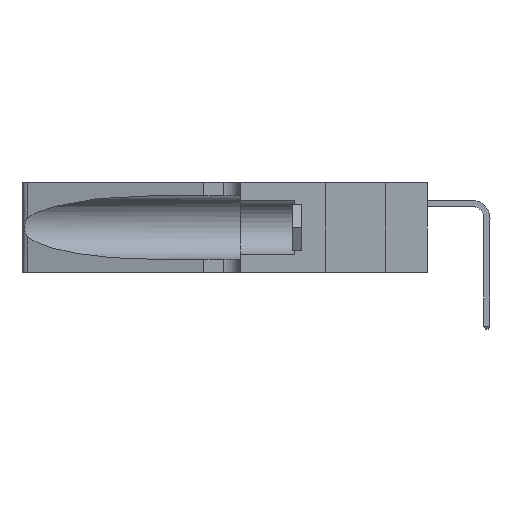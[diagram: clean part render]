
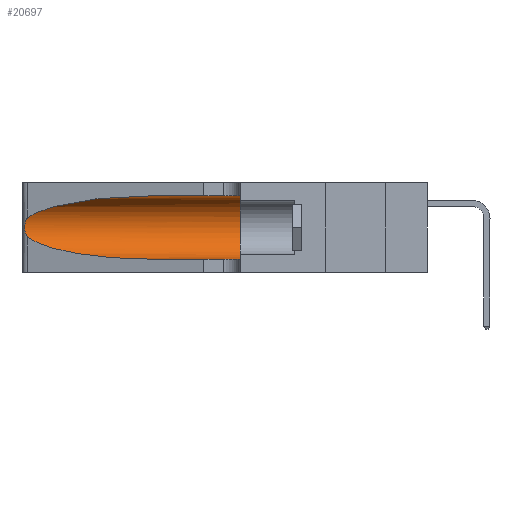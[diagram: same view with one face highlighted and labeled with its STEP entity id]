
A CAD part, left-side view. The second image highlights one B-rep face of the part: STEP entity #20697.
In plain terms, the highlighted cylindrical face has radius 3.308 mm (diameter 6.617 mm), a partial arc.
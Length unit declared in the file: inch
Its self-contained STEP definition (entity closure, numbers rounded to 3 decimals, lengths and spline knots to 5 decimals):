
#580 = VERTEX_POINT ( 'NONE', #30135 ) ;
#878 = VERTEX_POINT ( 'NONE', #23582 ) ;
#1025 = LINE ( 'NONE', #15702, #28114 ) ;
#1198 = DIRECTION ( 'NONE',  ( 0., 0., 1. ) ) ;
#1625 = CARTESIAN_POINT ( 'NONE',  ( 0.25787, 1.23484, 0.2124 ) ) ;
#4258 = CARTESIAN_POINT ( 'NONE',  ( 0.26018, 1.23835, 0.19895 ) ) ;
#4558 = CARTESIAN_POINT ( 'NONE',  ( 0.18966, 0.96281, 0.31525 ) ) ;
#4931 = EDGE_CURVE ( 'NONE', #878, #22970, #25974, .T. ) ;
#5900 = CIRCLE ( 'NONE', #28932, 0.13025 ) ;
#6622 = CYLINDRICAL_SURFACE ( 'NONE', #29486, 0.13025 ) ;
#6791 = CARTESIAN_POINT ( 'NONE',  ( 0.25555, 1.22994, 0.2215 ) ) ;
#6894 = CARTESIAN_POINT ( 'NONE',  ( 0.26075, 1.23896, 0.178 ) ) ;
#7195 = CARTESIAN_POINT ( 'NONE',  ( 0.2373, 1.15595, 0.28018 ) ) ;
#7427 = B_SPLINE_CURVE_WITH_KNOTS ( 'NONE', 3,
 ( #14649, #6791, #17309, #1625, #19964, #4258, #22632, #6894, #25282, #9506, #27890, #12143, #30555, #14763 ),
 .UNSPECIFIED., .F., .F.,
 ( 4, 2, 2, 2, 2, 2, 4 ),
 ( 0., 0.00027, 0.00053, 0.00107, 0.0016, 0.00187, 0.00214 ),
 .UNSPECIFIED. ) ;
#7447 = FACE_OUTER_BOUND ( 'NONE', #32667, .T. ) ;
#7489 = CARTESIAN_POINT ( 'NONE',  ( 0.2373, 1.15595, 0.08982 ) ) ;
#7947 = ORIENTED_EDGE ( 'NONE', *, *, #4931, .T. ) ;
#8421 = DIRECTION ( 'NONE',  ( 0., -1., 0. ) ) ;
#9506 = CARTESIAN_POINT ( 'NONE',  ( 0.25856, 1.23593, 0.16098 ) ) ;
#9768 = CARTESIAN_POINT ( 'NONE',  ( 0.1305, 1.61858, 0.185 ) ) ;
#10685 = CARTESIAN_POINT ( 'NONE',  ( 0.1305, 0.72297, 0.31525 ) ) ;
#12143 = CARTESIAN_POINT ( 'NONE',  ( 0.25639, 1.23186, 0.15144 ) ) ;
#12635 = CARTESIAN_POINT ( 'NONE',  ( 0.1305, 0.35, 0.31525 ) ) ;
#14649 = CARTESIAN_POINT ( 'NONE',  ( 0.25487, 1.22718, 0.22369 ) ) ;
#14763 = CARTESIAN_POINT ( 'NONE',  ( 0.25487, 1.22718, 0.14631 ) ) ;
#15386 = CARTESIAN_POINT ( 'NONE',  ( 0.1305, 0.72297, 0.05475 ) ) ;
#15601 = ORIENTED_EDGE ( 'NONE', *, *, #25103, .T. ) ;
#15702 = CARTESIAN_POINT ( 'NONE',  ( 0.1305, 1.61858, 0.31525 ) ) ;
#16545 = EDGE_CURVE ( 'NONE', #31386, #26524, #1025, .T. ) ;
#16882 = DIRECTION ( 'NONE',  ( 0., 1., 0. ) ) ;
#17309 = CARTESIAN_POINT ( 'NONE',  ( 0.25639, 1.23184, 0.21858 ) ) ;
#18256 = EDGE_CURVE ( 'NONE', #22970, #32600, #22673, .T. ) ;
#19964 = CARTESIAN_POINT ( 'NONE',  ( 0.25854, 1.2359, 0.20912 ) ) ;
#20272 = CARTESIAN_POINT ( 'NONE',  ( 0.1305, 0.72297, 0.31525 ) ) ;
#20697 = ADVANCED_FACE ( 'NONE', ( #7447 ), #6622, .F. ) ;
#22632 = CARTESIAN_POINT ( 'NONE',  ( 0.26075, 1.23896, 0.19203 ) ) ;
#22673 = LINE ( 'NONE', #24180, #30478 ) ;
#22970 = VERTEX_POINT ( 'NONE', #32320 ) ;
#23582 = CARTESIAN_POINT ( 'NONE',  ( 0.25487, 1.22718, 0.14631 ) ) ;
#24180 = CARTESIAN_POINT ( 'NONE',  ( 0.1305, 1.61858, 0.05475 ) ) ;
#24981 = ORIENTED_EDGE ( 'NONE', *, *, #27028, .T. ) ;
#25103 = EDGE_CURVE ( 'NONE', #31386, #580, #30370, .T. ) ;
#25282 = CARTESIAN_POINT ( 'NONE',  ( 0.26017, 1.23833, 0.17102 ) ) ;
#25534 = DIRECTION ( 'NONE',  ( 0., 0., -1. ) ) ;
#25561 = EDGE_CURVE ( 'NONE', #26524, #32600, #5900, .T. ) ;
#25581 = CARTESIAN_POINT ( 'NONE',  ( 0.25487, 1.22718, 0.22369 ) ) ;
#25974 =( BOUNDED_CURVE ( )  B_SPLINE_CURVE ( 3, ( #28376, #7489, #31142, #15386 ),
 .UNSPECIFIED., .F., .F. ) 
 B_SPLINE_CURVE_WITH_KNOTS ( ( 4, 4 ),
 ( 3.44316, 4.71239 ),
 .UNSPECIFIED. ) 
 CURVE ( )  GEOMETRIC_REPRESENTATION_ITEM ( )  RATIONAL_B_SPLINE_CURVE ( ( 1., 0.87, 0.87, 1. ) ) 
 REPRESENTATION_ITEM ( '' )  );
#26457 = CARTESIAN_POINT ( 'NONE',  ( 0.1305, 0.35, 0.05475 ) ) ;
#26524 = VERTEX_POINT ( 'NONE', #12635 ) ;
#26661 = ORIENTED_EDGE ( 'NONE', *, *, #16545, .F. ) ;
#27028 = EDGE_CURVE ( 'NONE', #580, #878, #7427, .T. ) ;
#27890 = CARTESIAN_POINT ( 'NONE',  ( 0.25789, 1.23486, 0.15765 ) ) ;
#28114 = VECTOR ( 'NONE', #28914, 39.37008 ) ;
#28376 = CARTESIAN_POINT ( 'NONE',  ( 0.25487, 1.22718, 0.14631 ) ) ;
#28610 = ORIENTED_EDGE ( 'NONE', *, *, #18256, .T. ) ;
#28914 = DIRECTION ( 'NONE',  ( 0., -1., 0. ) ) ;
#28932 = AXIS2_PLACEMENT_3D ( 'NONE', #32618, #16882, #1198 ) ;
#29486 = AXIS2_PLACEMENT_3D ( 'NONE', #9768, #30804, #25534 ) ;
#30135 = CARTESIAN_POINT ( 'NONE',  ( 0.25487, 1.22718, 0.22369 ) ) ;
#30370 =( BOUNDED_CURVE ( )  B_SPLINE_CURVE ( 3, ( #20272, #4558, #7195, #25581 ),
 .UNSPECIFIED., .F., .F. ) 
 B_SPLINE_CURVE_WITH_KNOTS ( ( 4, 4 ),
 ( 1.5708, 2.84003 ),
 .UNSPECIFIED. ) 
 CURVE ( )  GEOMETRIC_REPRESENTATION_ITEM ( )  RATIONAL_B_SPLINE_CURVE ( ( 1., 0.87, 0.87, 1. ) ) 
 REPRESENTATION_ITEM ( '' )  );
#30478 = VECTOR ( 'NONE', #8421, 39.37008 ) ;
#30555 = CARTESIAN_POINT ( 'NONE',  ( 0.25555, 1.22993, 0.14849 ) ) ;
#30804 = DIRECTION ( 'NONE',  ( 0., -1., 0. ) ) ;
#31142 = CARTESIAN_POINT ( 'NONE',  ( 0.18966, 0.96281, 0.05475 ) ) ;
#31386 = VERTEX_POINT ( 'NONE', #10685 ) ;
#32193 = ORIENTED_EDGE ( 'NONE', *, *, #25561, .F. ) ;
#32320 = CARTESIAN_POINT ( 'NONE',  ( 0.1305, 0.72297, 0.05475 ) ) ;
#32600 = VERTEX_POINT ( 'NONE', #26457 ) ;
#32618 = CARTESIAN_POINT ( 'NONE',  ( 0.1305, 0.35, 0.185 ) ) ;
#32667 = EDGE_LOOP ( 'NONE', ( #15601, #24981, #7947, #28610, #32193, #26661 ) ) ;
